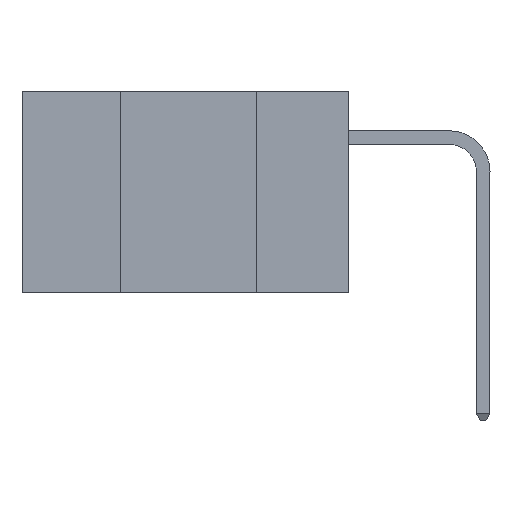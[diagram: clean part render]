
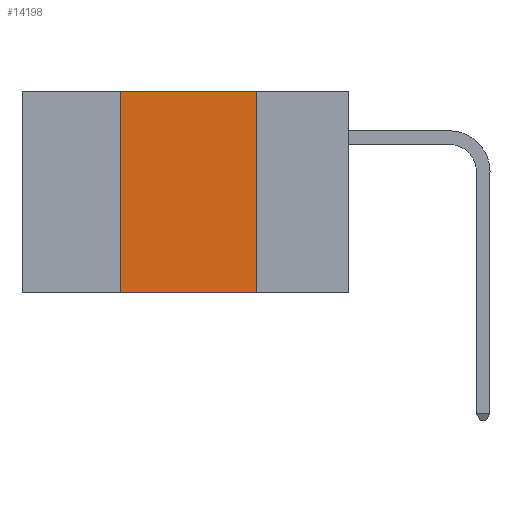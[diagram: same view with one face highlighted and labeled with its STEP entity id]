
A CAD part, left-side view. The second image highlights one B-rep face of the part: STEP entity #14198.
In plain terms, the highlighted planar face has unit normal (-1, 0, 0).
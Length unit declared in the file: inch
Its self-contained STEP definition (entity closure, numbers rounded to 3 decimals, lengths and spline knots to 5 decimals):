
#583 = CARTESIAN_POINT ( 'NONE',  ( 0., 0.17, -0.37 ) ) ;
#1263 = ORIENTED_EDGE ( 'NONE', *, *, #23513, .F. ) ;
#3637 = LINE ( 'NONE', #15939, #10466 ) ;
#4073 = LINE ( 'NONE', #16470, #26212 ) ;
#4743 = VECTOR ( 'NONE', #10017, 39.37008 ) ;
#5074 = DIRECTION ( 'NONE',  ( 0., 0., -1. ) ) ;
#6253 = LINE ( 'NONE', #8248, #7284 ) ;
#7257 = DIRECTION ( 'NONE',  ( 0., 0., -1. ) ) ;
#7284 = VECTOR ( 'NONE', #17388, 39.37008 ) ;
#8248 = CARTESIAN_POINT ( 'NONE',  ( 0., 0.42, 0. ) ) ;
#8853 = CARTESIAN_POINT ( 'NONE',  ( 0., 0.42, -0.37 ) ) ;
#8923 = FACE_OUTER_BOUND ( 'NONE', #17131, .T. ) ;
#9979 = AXIS2_PLACEMENT_3D ( 'NONE', #13812, #20460, #7257 ) ;
#10017 = DIRECTION ( 'NONE',  ( 0., -1., 0. ) ) ;
#10466 = VECTOR ( 'NONE', #5074, 39.37008 ) ;
#11908 = EDGE_CURVE ( 'NONE', #15094, #14681, #27555, .T. ) ;
#11992 = EDGE_CURVE ( 'NONE', #22803, #12232, #4073, .T. ) ;
#12232 = VERTEX_POINT ( 'NONE', #17595 ) ;
#13812 = CARTESIAN_POINT ( 'NONE',  ( 0., 0.6, 0. ) ) ;
#14198 = ADVANCED_FACE ( 'NONE', ( #8923 ), #18095, .F. ) ;
#14681 = VERTEX_POINT ( 'NONE', #583 ) ;
#15094 = VERTEX_POINT ( 'NONE', #8853 ) ;
#15939 = CARTESIAN_POINT ( 'NONE',  ( 0., 0.17, 0. ) ) ;
#16470 = CARTESIAN_POINT ( 'NONE',  ( 0., 0.6, 0. ) ) ;
#17131 = EDGE_LOOP ( 'NONE', ( #22099, #20548, #1263, #22066 ) ) ;
#17388 = DIRECTION ( 'NONE',  ( 0., 0., 1. ) ) ;
#17595 = CARTESIAN_POINT ( 'NONE',  ( 0., 0.17, 0. ) ) ;
#18020 = EDGE_CURVE ( 'NONE', #12232, #14681, #3637, .T. ) ;
#18095 = PLANE ( 'NONE',  #9979 ) ;
#20460 = DIRECTION ( 'NONE',  ( 1., 0., 0. ) ) ;
#20548 = ORIENTED_EDGE ( 'NONE', *, *, #11992, .F. ) ;
#22066 = ORIENTED_EDGE ( 'NONE', *, *, #11908, .T. ) ;
#22099 = ORIENTED_EDGE ( 'NONE', *, *, #18020, .F. ) ;
#22803 = VERTEX_POINT ( 'NONE', #23504 ) ;
#23035 = DIRECTION ( 'NONE',  ( 0., -1., 0. ) ) ;
#23405 = CARTESIAN_POINT ( 'NONE',  ( 0., 0.6, -0.37 ) ) ;
#23504 = CARTESIAN_POINT ( 'NONE',  ( 0., 0.42, 0. ) ) ;
#23513 = EDGE_CURVE ( 'NONE', #15094, #22803, #6253, .T. ) ;
#26212 = VECTOR ( 'NONE', #23035, 39.37008 ) ;
#27555 = LINE ( 'NONE', #23405, #4743 ) ;
